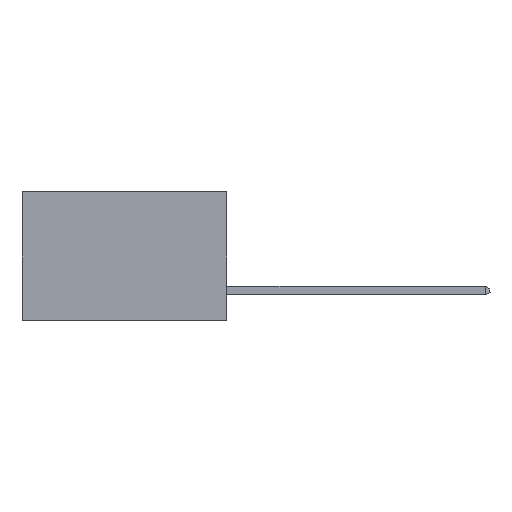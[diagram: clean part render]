
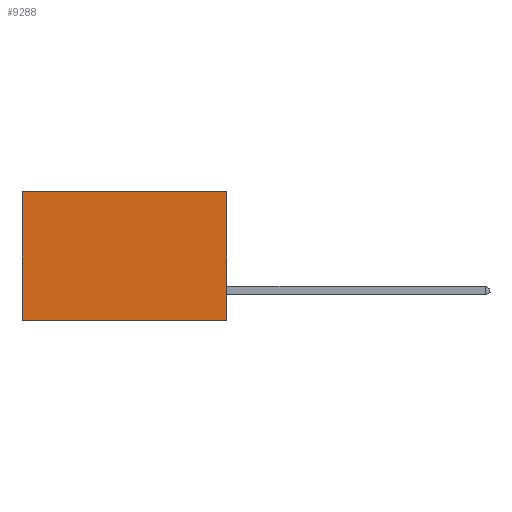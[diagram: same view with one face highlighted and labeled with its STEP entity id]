
A CAD part, left-side view. The second image highlights one B-rep face of the part: STEP entity #9288.
In plain terms, the highlighted planar face has unit normal (-1, 0, 0).
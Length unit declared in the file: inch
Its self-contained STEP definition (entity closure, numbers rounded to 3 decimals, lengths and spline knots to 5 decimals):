
#196 = CARTESIAN_POINT ( 'NONE',  ( 0.277, 0., 0. ) ) ;
#675 = DIRECTION ( 'NONE',  ( 0., 1., 0. ) ) ;
#682 = VECTOR ( 'NONE', #9625, 39.37008 ) ;
#1125 = CARTESIAN_POINT ( 'NONE',  ( 0.277, 0., -0.37 ) ) ;
#1198 = CARTESIAN_POINT ( 'NONE',  ( 0.277, 0.59, -0.37 ) ) ;
#1247 = LINE ( 'NONE', #3258, #5452 ) ;
#1618 = FACE_OUTER_BOUND ( 'NONE', #12668, .T. ) ;
#2013 = VERTEX_POINT ( 'NONE', #17840 ) ;
#2719 = DIRECTION ( 'NONE',  ( 1., 0., 0. ) ) ;
#2837 = ORIENTED_EDGE ( 'NONE', *, *, #13290, .F. ) ;
#2982 = CARTESIAN_POINT ( 'NONE',  ( 0.277, 0.59, 0. ) ) ;
#3258 = CARTESIAN_POINT ( 'NONE',  ( 0.277, 0., -0.37 ) ) ;
#3327 = DIRECTION ( 'NONE',  ( 0., 0., -1. ) ) ;
#3378 = LINE ( 'NONE', #10101, #19015 ) ;
#5452 = VECTOR ( 'NONE', #3327, 39.37008 ) ;
#5466 = ORIENTED_EDGE ( 'NONE', *, *, #6243, .F. ) ;
#6243 = EDGE_CURVE ( 'NONE', #12738, #8533, #1247, .T. ) ;
#6888 = CARTESIAN_POINT ( 'NONE',  ( 0.277, 0., 0. ) ) ;
#7672 = EDGE_CURVE ( 'NONE', #12738, #13061, #11760, .T. ) ;
#8199 = ORIENTED_EDGE ( 'NONE', *, *, #9313, .T. ) ;
#8533 = VERTEX_POINT ( 'NONE', #9934 ) ;
#9288 = ADVANCED_FACE ( 'NONE', ( #1618 ), #10548, .F. ) ;
#9313 = EDGE_CURVE ( 'NONE', #13061, #2013, #16980, .T. ) ;
#9625 = DIRECTION ( 'NONE',  ( 0., 1., 0. ) ) ;
#9934 = CARTESIAN_POINT ( 'NONE',  ( 0.277, 0., -0.37 ) ) ;
#10101 = CARTESIAN_POINT ( 'NONE',  ( 0.277, 0., -0.37 ) ) ;
#10548 = PLANE ( 'NONE',  #17542 ) ;
#11760 = LINE ( 'NONE', #196, #682 ) ;
#12172 = DIRECTION ( 'NONE',  ( 0., 0., -1. ) ) ;
#12668 = EDGE_LOOP ( 'NONE', ( #8199, #2837, #5466, #12916 ) ) ;
#12738 = VERTEX_POINT ( 'NONE', #6888 ) ;
#12916 = ORIENTED_EDGE ( 'NONE', *, *, #7672, .T. ) ;
#13061 = VERTEX_POINT ( 'NONE', #2982 ) ;
#13290 = EDGE_CURVE ( 'NONE', #8533, #2013, #3378, .T. ) ;
#13525 = VECTOR ( 'NONE', #12172, 39.37008 ) ;
#13572 = DIRECTION ( 'NONE',  ( 0., 0., -1. ) ) ;
#16980 = LINE ( 'NONE', #1198, #13525 ) ;
#17542 = AXIS2_PLACEMENT_3D ( 'NONE', #1125, #2719, #13572 ) ;
#17840 = CARTESIAN_POINT ( 'NONE',  ( 0.277, 0.59, -0.37 ) ) ;
#19015 = VECTOR ( 'NONE', #675, 39.37008 ) ;
